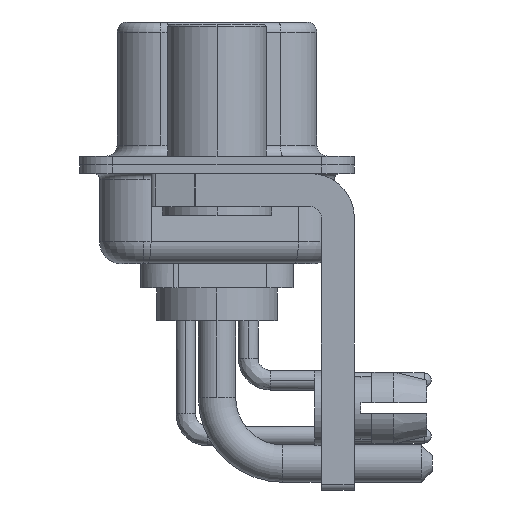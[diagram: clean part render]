
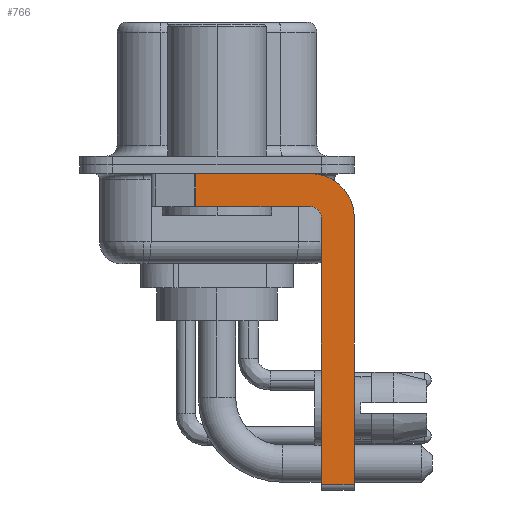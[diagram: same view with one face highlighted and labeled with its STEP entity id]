
A CAD part, left-side view. The second image highlights one B-rep face of the part: STEP entity #766.
In plain terms, the highlighted planar face has unit normal (-1, 0, 0).
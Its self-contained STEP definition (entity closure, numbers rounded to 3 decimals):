
#766 = ADVANCED_FACE ( 'NONE', ( #14327 ), #24222, .F. ) ;
#795 = EDGE_CURVE ( 'NONE', #29189, #20560, #5566, .T. ) ;
#1377 = ORIENTED_EDGE ( 'NONE', *, *, #29650, .F. ) ;
#1984 = CARTESIAN_POINT ( 'NONE',  ( -2.9, -4.25, -2.4 ) ) ;
#2332 = CARTESIAN_POINT ( 'NONE',  ( -2.9, 0.978, -0.4 ) ) ;
#3064 = CARTESIAN_POINT ( 'NONE',  ( -2.9, -6.25, -2.4 ) ) ;
#3769 = VECTOR ( 'NONE', #15248, 1000. ) ;
#4119 = VECTOR ( 'NONE', #30000, 1000. ) ;
#4836 = CARTESIAN_POINT ( 'NONE',  ( -2.9, -4.25, -1.9 ) ) ;
#5320 = DIRECTION ( 'NONE',  ( 0., 1., 0. ) ) ;
#5566 = LINE ( 'NONE', #17557, #16673 ) ;
#5632 = DIRECTION ( 'NONE',  ( -1., 0., 0. ) ) ;
#6459 = VERTEX_POINT ( 'NONE', #27985 ) ;
#6503 = VERTEX_POINT ( 'NONE', #15337 ) ;
#7387 = EDGE_LOOP ( 'NONE', ( #29515, #30735, #22163, #20088, #29677, #31774, #24467, #1377 ) ) ;
#7502 = CARTESIAN_POINT ( 'NONE',  ( -2.9, -6.25, -2.4 ) ) ;
#8079 = CARTESIAN_POINT ( 'NONE',  ( -2.9, -4.25, -2.4 ) ) ;
#9856 = DIRECTION ( 'NONE',  ( 0., 0., -1. ) ) ;
#10400 = CARTESIAN_POINT ( 'NONE',  ( -2.9, 0.978, -1.9 ) ) ;
#10917 = LINE ( 'NONE', #3064, #4119 ) ;
#10965 = CIRCLE ( 'NONE', #13061, 2. ) ;
#11257 = DIRECTION ( 'NONE',  ( 0., 0., 1. ) ) ;
#11899 = DIRECTION ( 'NONE',  ( 1., 0., 0. ) ) ;
#12079 = VERTEX_POINT ( 'NONE', #31237 ) ;
#12277 = DIRECTION ( 'NONE',  ( 1., 0., 0. ) ) ;
#12288 = LINE ( 'NONE', #4836, #17920 ) ;
#12540 = CARTESIAN_POINT ( 'NONE',  ( -2.9, -4.75, -14.55 ) ) ;
#12634 = VERTEX_POINT ( 'NONE', #7502 ) ;
#13061 = AXIS2_PLACEMENT_3D ( 'NONE', #27197, #12277, #9856 ) ;
#13344 = DIRECTION ( 'NONE',  ( 0., -1., 0. ) ) ;
#14327 = FACE_OUTER_BOUND ( 'NONE', #7387, .T. ) ;
#14575 = EDGE_CURVE ( 'NONE', #12079, #20040, #20763, .T. ) ;
#15248 = DIRECTION ( 'NONE',  ( 0., 0., -1. ) ) ;
#15337 = CARTESIAN_POINT ( 'NONE',  ( -2.9, 0.978, -1.9 ) ) ;
#15672 = LINE ( 'NONE', #20224, #18890 ) ;
#16673 = VECTOR ( 'NONE', #13344, 1000. ) ;
#16961 = VECTOR ( 'NONE', #19917, 1000. ) ;
#17557 = CARTESIAN_POINT ( 'NONE',  ( -2.9, 3., -0.4 ) ) ;
#17652 = EDGE_CURVE ( 'NONE', #29189, #6503, #25470, .T. ) ;
#17920 = VECTOR ( 'NONE', #5320, 1000. ) ;
#18890 = VECTOR ( 'NONE', #30118, 1000. ) ;
#19917 = DIRECTION ( 'NONE',  ( 0., 0., 1. ) ) ;
#20040 = VERTEX_POINT ( 'NONE', #29239 ) ;
#20079 = VERTEX_POINT ( 'NONE', #12540 ) ;
#20088 = ORIENTED_EDGE ( 'NONE', *, *, #14575, .F. ) ;
#20224 = CARTESIAN_POINT ( 'NONE',  ( -2.9, -4.25, -14.55 ) ) ;
#20560 = VERTEX_POINT ( 'NONE', #27248 ) ;
#20763 = CIRCLE ( 'NONE', #29056, 0.5 ) ;
#21038 = EDGE_CURVE ( 'NONE', #20040, #6503, #12288, .T. ) ;
#21231 = EDGE_CURVE ( 'NONE', #20079, #6459, #15672, .T. ) ;
#21788 = DIRECTION ( 'NONE',  ( 0., 0., -1. ) ) ;
#22163 = ORIENTED_EDGE ( 'NONE', *, *, #21038, .F. ) ;
#23955 = AXIS2_PLACEMENT_3D ( 'NONE', #1984, #11899, #21788 ) ;
#24222 = PLANE ( 'NONE',  #23955 ) ;
#24467 = ORIENTED_EDGE ( 'NONE', *, *, #28126, .F. ) ;
#25470 = LINE ( 'NONE', #10400, #3769 ) ;
#25634 = EDGE_CURVE ( 'NONE', #20079, #12079, #27060, .T. ) ;
#27060 = LINE ( 'NONE', #29648, #16961 ) ;
#27197 = CARTESIAN_POINT ( 'NONE',  ( -2.9, -4.25, -2.4 ) ) ;
#27248 = CARTESIAN_POINT ( 'NONE',  ( -2.9, -4.25, -0.4 ) ) ;
#27985 = CARTESIAN_POINT ( 'NONE',  ( -2.9, -6.25, -14.55 ) ) ;
#28126 = EDGE_CURVE ( 'NONE', #12634, #6459, #10917, .T. ) ;
#29056 = AXIS2_PLACEMENT_3D ( 'NONE', #8079, #5632, #11257 ) ;
#29189 = VERTEX_POINT ( 'NONE', #2332 ) ;
#29239 = CARTESIAN_POINT ( 'NONE',  ( -2.9, -4.25, -1.9 ) ) ;
#29515 = ORIENTED_EDGE ( 'NONE', *, *, #795, .F. ) ;
#29648 = CARTESIAN_POINT ( 'NONE',  ( -2.9, -4.75, -14.8 ) ) ;
#29650 = EDGE_CURVE ( 'NONE', #20560, #12634, #10965, .T. ) ;
#29677 = ORIENTED_EDGE ( 'NONE', *, *, #25634, .F. ) ;
#30000 = DIRECTION ( 'NONE',  ( 0., 0., -1. ) ) ;
#30118 = DIRECTION ( 'NONE',  ( 0., -1., 0. ) ) ;
#30735 = ORIENTED_EDGE ( 'NONE', *, *, #17652, .T. ) ;
#31237 = CARTESIAN_POINT ( 'NONE',  ( -2.9, -4.75, -2.4 ) ) ;
#31774 = ORIENTED_EDGE ( 'NONE', *, *, #21231, .T. ) ;
